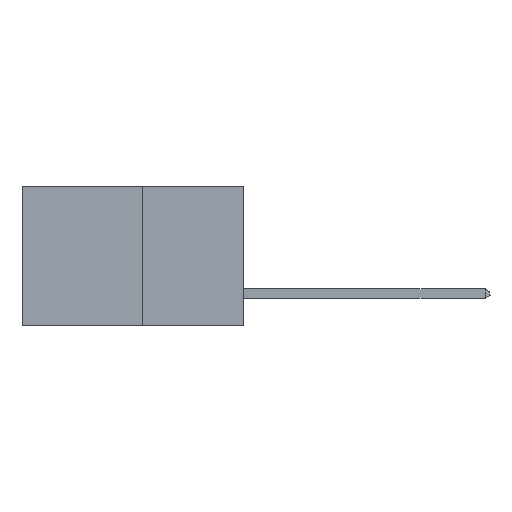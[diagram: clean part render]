
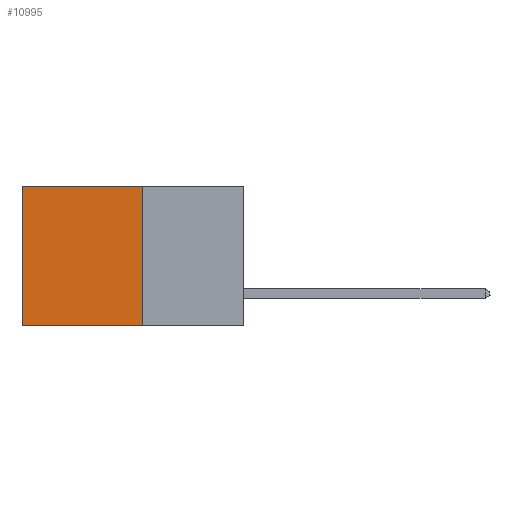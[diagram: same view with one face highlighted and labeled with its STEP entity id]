
A CAD part, left-side view. The second image highlights one B-rep face of the part: STEP entity #10995.
In plain terms, the highlighted planar face has unit normal (-1, 0, 0).
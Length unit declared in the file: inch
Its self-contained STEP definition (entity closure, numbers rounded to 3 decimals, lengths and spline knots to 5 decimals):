
#482 = DIRECTION ( 'NONE',  ( 0., 1., 0. ) ) ;
#964 = ORIENTED_EDGE ( 'NONE', *, *, #11141, .T. ) ;
#1019 = AXIS2_PLACEMENT_3D ( 'NONE', #10081, #11986, #6181 ) ;
#1122 = VERTEX_POINT ( 'NONE', #11108 ) ;
#1252 = PLANE ( 'NONE',  #1019 ) ;
#1271 = CARTESIAN_POINT ( 'NONE',  ( 0.277, 0.27, -0.37 ) ) ;
#1623 = ORIENTED_EDGE ( 'NONE', *, *, #7397, .F. ) ;
#1805 = LINE ( 'NONE', #2947, #9321 ) ;
#2390 = VERTEX_POINT ( 'NONE', #6521 ) ;
#2947 = CARTESIAN_POINT ( 'NONE',  ( 0.277, 0.59, -0.37 ) ) ;
#2971 = CARTESIAN_POINT ( 'NONE',  ( 0.277, 0.59, 0. ) ) ;
#3110 = VECTOR ( 'NONE', #482, 39.37008 ) ;
#3693 = VECTOR ( 'NONE', #11998, 39.37008 ) ;
#3937 = DIRECTION ( 'NONE',  ( 0., 0., -1. ) ) ;
#4158 = FACE_OUTER_BOUND ( 'NONE', #6834, .T. ) ;
#4907 = VECTOR ( 'NONE', #6384, 39.37008 ) ;
#6181 = DIRECTION ( 'NONE',  ( 0., 0., -1. ) ) ;
#6384 = DIRECTION ( 'NONE',  ( 0., 1., 0. ) ) ;
#6521 = CARTESIAN_POINT ( 'NONE',  ( 0.277, 0.27, 0. ) ) ;
#6834 = EDGE_LOOP ( 'NONE', ( #11052, #1623, #9515, #964 ) ) ;
#6836 = CARTESIAN_POINT ( 'NONE',  ( 0.277, 0.27, -0.37 ) ) ;
#7044 = EDGE_CURVE ( 'NONE', #10330, #1122, #1805, .T. ) ;
#7381 = CARTESIAN_POINT ( 'NONE',  ( 0.277, 0.27, 0. ) ) ;
#7397 = EDGE_CURVE ( 'NONE', #9084, #1122, #10878, .T. ) ;
#9084 = VERTEX_POINT ( 'NONE', #6836 ) ;
#9299 = EDGE_CURVE ( 'NONE', #2390, #9084, #11732, .T. ) ;
#9321 = VECTOR ( 'NONE', #3937, 39.37008 ) ;
#9515 = ORIENTED_EDGE ( 'NONE', *, *, #9299, .F. ) ;
#10081 = CARTESIAN_POINT ( 'NONE',  ( 0.277, 0.27, -0.37 ) ) ;
#10093 = LINE ( 'NONE', #7381, #4907 ) ;
#10330 = VERTEX_POINT ( 'NONE', #2971 ) ;
#10878 = LINE ( 'NONE', #11245, #3110 ) ;
#10995 = ADVANCED_FACE ( 'NONE', ( #4158 ), #1252, .F. ) ;
#11052 = ORIENTED_EDGE ( 'NONE', *, *, #7044, .T. ) ;
#11108 = CARTESIAN_POINT ( 'NONE',  ( 0.277, 0.59, -0.37 ) ) ;
#11141 = EDGE_CURVE ( 'NONE', #2390, #10330, #10093, .T. ) ;
#11245 = CARTESIAN_POINT ( 'NONE',  ( 0.277, 0.27, -0.37 ) ) ;
#11732 = LINE ( 'NONE', #1271, #3693 ) ;
#11986 = DIRECTION ( 'NONE',  ( 1., 0., 0. ) ) ;
#11998 = DIRECTION ( 'NONE',  ( 0., 0., -1. ) ) ;
